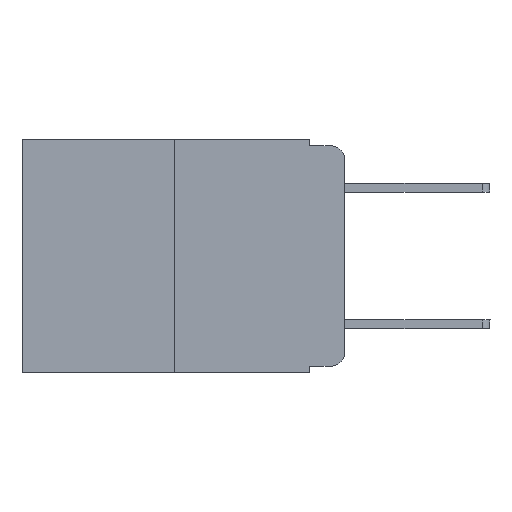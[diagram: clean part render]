
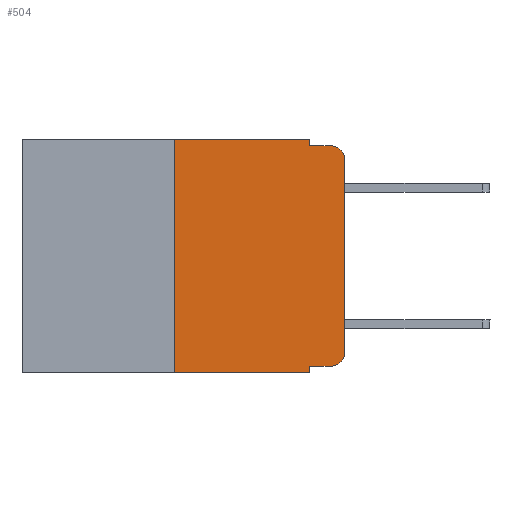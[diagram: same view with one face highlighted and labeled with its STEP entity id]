
A CAD part, left-side view. The second image highlights one B-rep face of the part: STEP entity #504.
In plain terms, the highlighted planar face has unit normal (-1, 0, 0).
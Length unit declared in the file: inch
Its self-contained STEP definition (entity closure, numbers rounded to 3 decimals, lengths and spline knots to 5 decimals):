
#54 = DIRECTION ( 'NONE',  ( 0., 0., -1. ) ) ;
#504 = ADVANCED_FACE ( 'NONE', ( #1581 ), #8534, .F. ) ;
#810 = VERTEX_POINT ( 'NONE', #10379 ) ;
#1181 = EDGE_CURVE ( 'NONE', #22215, #12493, #3462, .T. ) ;
#1361 = AXIS2_PLACEMENT_3D ( 'NONE', #12393, #8872, #9651 ) ;
#1496 = EDGE_CURVE ( 'NONE', #14736, #18588, #18244, .T. ) ;
#1581 = FACE_OUTER_BOUND ( 'NONE', #17692, .T. ) ;
#1871 = EDGE_CURVE ( 'NONE', #19760, #12182, #12860, .T. ) ;
#2019 = CARTESIAN_POINT ( 'NONE',  ( 0., 0.02, -0.01 ) ) ;
#2021 = CARTESIAN_POINT ( 'NONE',  ( 0., 0.051, 0. ) ) ;
#2066 = EDGE_CURVE ( 'NONE', #12260, #810, #15760, .T. ) ;
#2896 = CARTESIAN_POINT ( 'NONE',  ( 0., 0.473, 0. ) ) ;
#3130 = LINE ( 'NONE', #16965, #13536 ) ;
#3462 = LINE ( 'NONE', #10407, #18208 ) ;
#3512 = CIRCLE ( 'NONE', #16190, 0.02 ) ;
#4060 = CIRCLE ( 'NONE', #17464, 0.02 ) ;
#4387 = VECTOR ( 'NONE', #17251, 39.37008 ) ;
#4764 = ORIENTED_EDGE ( 'NONE', *, *, #1871, .T. ) ;
#5050 = VECTOR ( 'NONE', #9022, 39.37008 ) ;
#5060 = DIRECTION ( 'NONE',  ( 0., 0., 1. ) ) ;
#5186 = CARTESIAN_POINT ( 'NONE',  ( 0., 0.02, -0.03 ) ) ;
#5224 = CARTESIAN_POINT ( 'NONE',  ( 0., 0., -0.313 ) ) ;
#5430 = DIRECTION ( 'NONE',  ( -1., 0., 0. ) ) ;
#5953 = EDGE_CURVE ( 'NONE', #15095, #19760, #4060, .T. ) ;
#6083 = ORIENTED_EDGE ( 'NONE', *, *, #7979, .F. ) ;
#6194 = ORIENTED_EDGE ( 'NONE', *, *, #22294, .T. ) ;
#6950 = VECTOR ( 'NONE', #14569, 39.37008 ) ;
#7183 = EDGE_CURVE ( 'NONE', #12260, #14736, #3130, .T. ) ;
#7979 = EDGE_CURVE ( 'NONE', #14851, #810, #20003, .T. ) ;
#8349 = ORIENTED_EDGE ( 'NONE', *, *, #1496, .F. ) ;
#8534 = PLANE ( 'NONE',  #1361 ) ;
#8872 = DIRECTION ( 'NONE',  ( 1., 0., 0. ) ) ;
#9022 = DIRECTION ( 'NONE',  ( 0., -1., 0. ) ) ;
#9651 = DIRECTION ( 'NONE',  ( 0., 0., -1. ) ) ;
#9677 = CARTESIAN_POINT ( 'NONE',  ( 0., 0., 0. ) ) ;
#10379 = CARTESIAN_POINT ( 'NONE',  ( 0., 0.051, -0.343 ) ) ;
#10407 = CARTESIAN_POINT ( 'NONE',  ( 0., 0.051, -0.01 ) ) ;
#10729 = LINE ( 'NONE', #16028, #5050 ) ;
#11141 = CARTESIAN_POINT ( 'NONE',  ( 0., 0.051, 0. ) ) ;
#12042 = CARTESIAN_POINT ( 'NONE',  ( 0., 0.051, 0. ) ) ;
#12131 = ORIENTED_EDGE ( 'NONE', *, *, #16343, .T. ) ;
#12180 = DIRECTION ( 'NONE',  ( -1., 0., 0. ) ) ;
#12182 = VERTEX_POINT ( 'NONE', #16277 ) ;
#12260 = VERTEX_POINT ( 'NONE', #17891 ) ;
#12393 = CARTESIAN_POINT ( 'NONE',  ( 0., 0.473, 0. ) ) ;
#12475 = ORIENTED_EDGE ( 'NONE', *, *, #7183, .F. ) ;
#12493 = VERTEX_POINT ( 'NONE', #2019 ) ;
#12860 = LINE ( 'NONE', #9677, #18013 ) ;
#13519 = ORIENTED_EDGE ( 'NONE', *, *, #17064, .F. ) ;
#13536 = VECTOR ( 'NONE', #5060, 39.37008 ) ;
#13861 = VECTOR ( 'NONE', #21218, 39.37008 ) ;
#13904 = CARTESIAN_POINT ( 'NONE',  ( 0., 0.25, 0. ) ) ;
#14569 = DIRECTION ( 'NONE',  ( 0., -1., 0. ) ) ;
#14605 = ORIENTED_EDGE ( 'NONE', *, *, #2066, .T. ) ;
#14736 = VERTEX_POINT ( 'NONE', #13904 ) ;
#14851 = VERTEX_POINT ( 'NONE', #16283 ) ;
#15095 = VERTEX_POINT ( 'NONE', #19132 ) ;
#15559 = DIRECTION ( 'NONE',  ( 0., 0., -1. ) ) ;
#15760 = LINE ( 'NONE', #17489, #13861 ) ;
#16028 = CARTESIAN_POINT ( 'NONE',  ( 0., 0.051, -0.333 ) ) ;
#16190 = AXIS2_PLACEMENT_3D ( 'NONE', #5186, #5430, #54 ) ;
#16277 = CARTESIAN_POINT ( 'NONE',  ( 0., 0., -0.03 ) ) ;
#16283 = CARTESIAN_POINT ( 'NONE',  ( 0., 0.051, -0.333 ) ) ;
#16343 = EDGE_CURVE ( 'NONE', #14851, #15095, #10729, .T. ) ;
#16371 = ORIENTED_EDGE ( 'NONE', *, *, #5953, .T. ) ;
#16393 = VECTOR ( 'NONE', #19771, 39.37008 ) ;
#16965 = CARTESIAN_POINT ( 'NONE',  ( 0., 0.25, 0. ) ) ;
#17064 = EDGE_CURVE ( 'NONE', #18588, #22215, #22019, .T. ) ;
#17251 = DIRECTION ( 'NONE',  ( 0., 0., -1. ) ) ;
#17417 = DIRECTION ( 'NONE',  ( 0., -1., 0. ) ) ;
#17464 = AXIS2_PLACEMENT_3D ( 'NONE', #19109, #12180, #15559 ) ;
#17489 = CARTESIAN_POINT ( 'NONE',  ( 0., 0.473, -0.343 ) ) ;
#17692 = EDGE_LOOP ( 'NONE', ( #4764, #6194, #22387, #13519, #8349, #12475, #14605, #6083, #12131, #16371 ) ) ;
#17891 = CARTESIAN_POINT ( 'NONE',  ( 0., 0.25, -0.343 ) ) ;
#18013 = VECTOR ( 'NONE', #19796, 39.37008 ) ;
#18208 = VECTOR ( 'NONE', #17417, 39.37008 ) ;
#18244 = LINE ( 'NONE', #2896, #6950 ) ;
#18588 = VERTEX_POINT ( 'NONE', #2021 ) ;
#19109 = CARTESIAN_POINT ( 'NONE',  ( 0., 0.02, -0.313 ) ) ;
#19132 = CARTESIAN_POINT ( 'NONE',  ( 0., 0.02, -0.333 ) ) ;
#19760 = VERTEX_POINT ( 'NONE', #5224 ) ;
#19771 = DIRECTION ( 'NONE',  ( 0., 0., -1. ) ) ;
#19796 = DIRECTION ( 'NONE',  ( 0., 0., 1. ) ) ;
#20003 = LINE ( 'NONE', #11141, #16393 ) ;
#21218 = DIRECTION ( 'NONE',  ( 0., -1., 0. ) ) ;
#22019 = LINE ( 'NONE', #12042, #4387 ) ;
#22092 = CARTESIAN_POINT ( 'NONE',  ( 0., 0.051, -0.01 ) ) ;
#22215 = VERTEX_POINT ( 'NONE', #22092 ) ;
#22294 = EDGE_CURVE ( 'NONE', #12182, #12493, #3512, .T. ) ;
#22387 = ORIENTED_EDGE ( 'NONE', *, *, #1181, .F. ) ;
